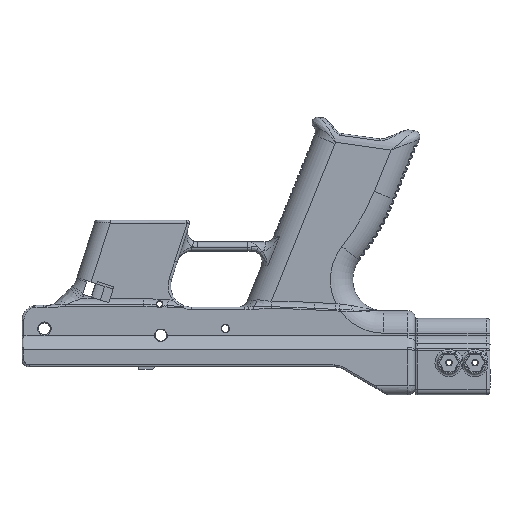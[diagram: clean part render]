
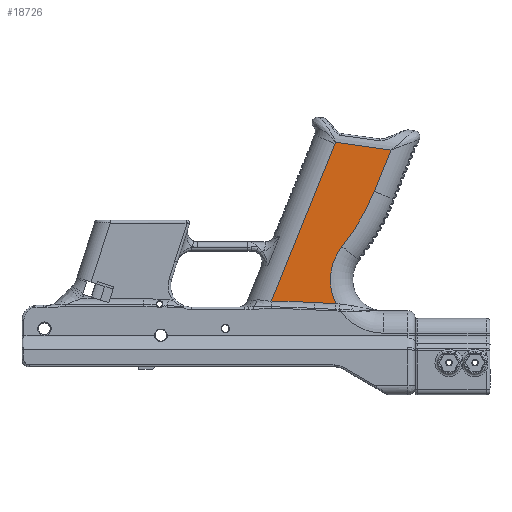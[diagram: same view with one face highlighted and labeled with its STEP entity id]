
A CAD part, front view. The second image highlights one B-rep face of the part: STEP entity #18726.
In plain terms, the highlighted planar face has unit normal (0, -1, 0).
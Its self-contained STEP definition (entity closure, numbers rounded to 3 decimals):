
#2033=CIRCLE('',#19939,118.894);
#2421=CIRCLE('',#20696,689.416);
#2423=CIRCLE('',#20699,696.304);
#2438=CIRCLE('',#20722,28.63);
#2439=CIRCLE('',#20723,17.);
#3923=FACE_OUTER_BOUND('',#5136,.T.);
#5136=EDGE_LOOP('',(#17211,#17212,#17213,#17214,#17215,#17216,#17217,#17218));
#5482=LINE('',#28979,#6492);
#5731=LINE('',#39514,#6741);
#6160=LINE('',#47972,#7170);
#6492=VECTOR('',#22074,10.);
#6741=VECTOR('',#23643,10.);
#7170=VECTOR('',#25666,10.);
#7616=VERTEX_POINT('',#28976);
#7617=VERTEX_POINT('',#28978);
#8156=VERTEX_POINT('',#39506);
#8157=VERTEX_POINT('',#39513);
#8158=VERTEX_POINT('',#39530);
#8813=VERTEX_POINT('',#47523);
#8814=VERTEX_POINT('',#47530);
#8821=VERTEX_POINT('',#47971);
#9514=EDGE_CURVE('',#7616,#7617,#5482,.T.);
#10445=EDGE_CURVE('',#8156,#8157,#5731,.T.);
#10449=EDGE_CURVE('',#7617,#8158,#2033,.T.);
#11605=EDGE_CURVE('',#8813,#8814,#2421,.T.);
#11607=EDGE_CURVE('',#8814,#8156,#2423,.T.);
#11629=EDGE_CURVE('',#8158,#8813,#2438,.T.);
#11630=EDGE_CURVE('',#8821,#7616,#6160,.T.);
#11631=EDGE_CURVE('',#8157,#8821,#2439,.T.);
#17211=ORIENTED_EDGE('',*,*,#11605,.F.);
#17212=ORIENTED_EDGE('',*,*,#11629,.F.);
#17213=ORIENTED_EDGE('',*,*,#10449,.F.);
#17214=ORIENTED_EDGE('',*,*,#9514,.F.);
#17215=ORIENTED_EDGE('',*,*,#11630,.F.);
#17216=ORIENTED_EDGE('',*,*,#11631,.F.);
#17217=ORIENTED_EDGE('',*,*,#10445,.F.);
#17218=ORIENTED_EDGE('',*,*,#11607,.F.);
#17571=PLANE('',#20721);
#18726=ADVANCED_FACE('',(#3923),#17571,.T.);
#19939=AXIS2_PLACEMENT_3D('',#39531,#23672,#23673);
#20696=AXIS2_PLACEMENT_3D('',#47531,#25612,#25613);
#20699=AXIS2_PLACEMENT_3D('',#47534,#25618,#25619);
#20721=AXIS2_PLACEMENT_3D('',#47969,#25662,#25663);
#20722=AXIS2_PLACEMENT_3D('',#47970,#25664,#25665);
#20723=AXIS2_PLACEMENT_3D('',#47973,#25667,#25668);
#22074=DIRECTION('',(-0.375,0.,-0.927));
#23643=DIRECTION('',(0.375,0.,0.927));
#23672=DIRECTION('center_axis',(0.,1.,0.));
#23673=DIRECTION('ref_axis',(0.891,0.,-0.454));
#25612=DIRECTION('center_axis',(0.,1.,0.));
#25613=DIRECTION('ref_axis',(0.037,0.,0.999));
#25618=DIRECTION('center_axis',(0.,-1.,0.));
#25619=DIRECTION('ref_axis',(-0.054,0.,-0.999));
#25662=DIRECTION('center_axis',(0.,-1.,0.));
#25663=DIRECTION('ref_axis',(1.,0.,0.));
#25664=DIRECTION('center_axis',(0.,-1.,0.));
#25665=DIRECTION('ref_axis',(0.782,0.,-0.624));
#25666=DIRECTION('',(0.99,0.,-0.139));
#25667=DIRECTION('center_axis',(0.,-1.,0.));
#25668=DIRECTION('ref_axis',(0.992,0.,0.126));
#28976=CARTESIAN_POINT('',(117.841,-14.625,19.236));
#28978=CARTESIAN_POINT('',(108.893,-14.625,-2.912));
#28979=CARTESIAN_POINT('',(111.761,-14.625,4.188));
#39506=CARTESIAN_POINT('',(53.832,-14.625,-61.703));
#39513=CARTESIAN_POINT('',(87.937,-14.625,22.71));
#39514=CARTESIAN_POINT('',(70.22,-14.625,-21.141));
#39530=CARTESIAN_POINT('',(91.6,-14.625,-32.517));
#39531=CARTESIAN_POINT('Origin',(-1.344,-14.625,41.627));
#47523=CARTESIAN_POINT('',(88.326,-14.625,-63.079));
#47530=CARTESIAN_POINT('',(76.954,-14.625,-62.561));
#47531=CARTESIAN_POINT('Origin',(113.981,-14.625,625.86));
#47534=CARTESIAN_POINT('Origin',(39.557,-14.625,-757.86));
#47969=CARTESIAN_POINT('Origin',(86.464,-14.625,-15.081));
#47970=CARTESIAN_POINT('Origin',(113.981,-14.625,-50.37));
#47971=CARTESIAN_POINT('',(88.199,-14.625,23.402));
#47972=CARTESIAN_POINT('',(84.577,-14.625,23.911));
#47973=CARTESIAN_POINT('Origin',(72.175,-14.625,29.078));
